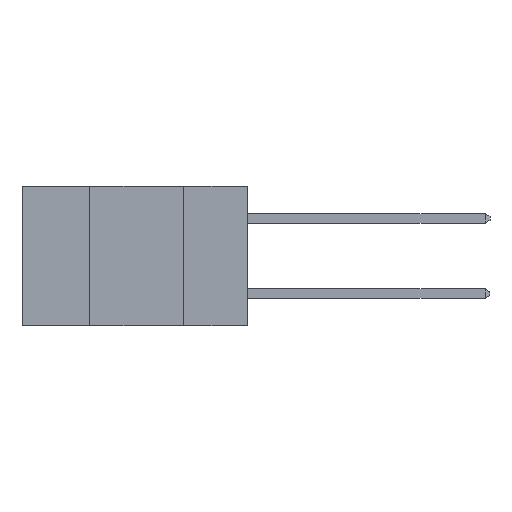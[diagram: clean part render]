
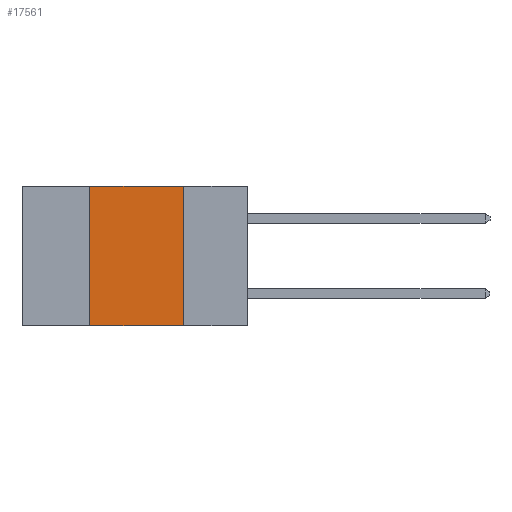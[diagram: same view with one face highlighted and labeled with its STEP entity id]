
A CAD part, left-side view. The second image highlights one B-rep face of the part: STEP entity #17561.
In plain terms, the highlighted planar face has unit normal (-1, 0, 0).
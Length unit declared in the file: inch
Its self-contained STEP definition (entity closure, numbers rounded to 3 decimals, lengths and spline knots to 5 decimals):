
#178 = LINE ( 'NONE', #14852, #16578 ) ;
#222 = LINE ( 'NONE', #686, #11452 ) ;
#263 = EDGE_CURVE ( 'NONE', #4351, #11520, #222, .T. ) ;
#536 = VECTOR ( 'NONE', #14584, 39.37008 ) ;
#537 = EDGE_LOOP ( 'NONE', ( #8967, #9332, #3083, #7066 ) ) ;
#686 = CARTESIAN_POINT ( 'NONE',  ( 0., 0.17, 0. ) ) ;
#1692 = AXIS2_PLACEMENT_3D ( 'NONE', #17957, #8681, #19483 ) ;
#1981 = VERTEX_POINT ( 'NONE', #12403 ) ;
#3083 = ORIENTED_EDGE ( 'NONE', *, *, #14540, .F. ) ;
#4351 = VERTEX_POINT ( 'NONE', #13925 ) ;
#5466 = DIRECTION ( 'NONE',  ( 0., 0., 1. ) ) ;
#7066 = ORIENTED_EDGE ( 'NONE', *, *, #10316, .T. ) ;
#8432 = CARTESIAN_POINT ( 'NONE',  ( 0., 0.17, -0.37 ) ) ;
#8681 = DIRECTION ( 'NONE',  ( 1., 0., 0. ) ) ;
#8777 = VECTOR ( 'NONE', #9944, 39.37008 ) ;
#8967 = ORIENTED_EDGE ( 'NONE', *, *, #263, .F. ) ;
#9332 = ORIENTED_EDGE ( 'NONE', *, *, #17770, .F. ) ;
#9944 = DIRECTION ( 'NONE',  ( 0., -1., 0. ) ) ;
#10316 = EDGE_CURVE ( 'NONE', #15317, #11520, #17515, .T. ) ;
#11117 = CARTESIAN_POINT ( 'NONE',  ( 0., 0.42, -0.37 ) ) ;
#11452 = VECTOR ( 'NONE', #13252, 39.37008 ) ;
#11520 = VERTEX_POINT ( 'NONE', #8432 ) ;
#11729 = PLANE ( 'NONE',  #1692 ) ;
#12403 = CARTESIAN_POINT ( 'NONE',  ( 0., 0.42, 0. ) ) ;
#12762 = LINE ( 'NONE', #19111, #536 ) ;
#13252 = DIRECTION ( 'NONE',  ( 0., 0., -1. ) ) ;
#13925 = CARTESIAN_POINT ( 'NONE',  ( 0., 0.17, 0. ) ) ;
#14540 = EDGE_CURVE ( 'NONE', #15317, #1981, #178, .T. ) ;
#14584 = DIRECTION ( 'NONE',  ( 0., -1., 0. ) ) ;
#14852 = CARTESIAN_POINT ( 'NONE',  ( 0., 0.42, 0. ) ) ;
#15317 = VERTEX_POINT ( 'NONE', #11117 ) ;
#16201 = FACE_OUTER_BOUND ( 'NONE', #537, .T. ) ;
#16207 = CARTESIAN_POINT ( 'NONE',  ( 0., 0.6, -0.37 ) ) ;
#16578 = VECTOR ( 'NONE', #5466, 39.37008 ) ;
#17515 = LINE ( 'NONE', #16207, #8777 ) ;
#17561 = ADVANCED_FACE ( 'NONE', ( #16201 ), #11729, .F. ) ;
#17770 = EDGE_CURVE ( 'NONE', #1981, #4351, #12762, .T. ) ;
#17957 = CARTESIAN_POINT ( 'NONE',  ( 0., 0.6, 0. ) ) ;
#19111 = CARTESIAN_POINT ( 'NONE',  ( 0., 0.6, 0. ) ) ;
#19483 = DIRECTION ( 'NONE',  ( 0., 0., -1. ) ) ;
